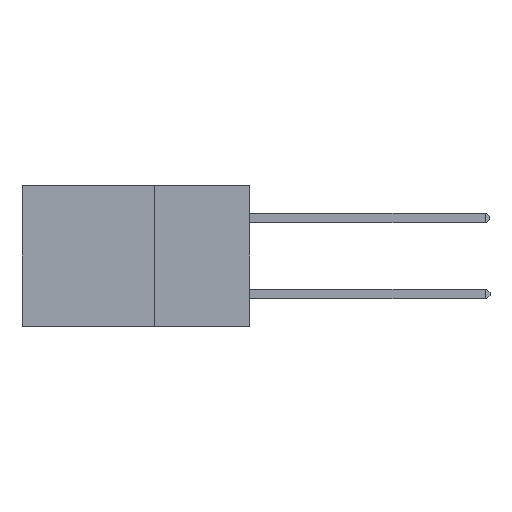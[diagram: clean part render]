
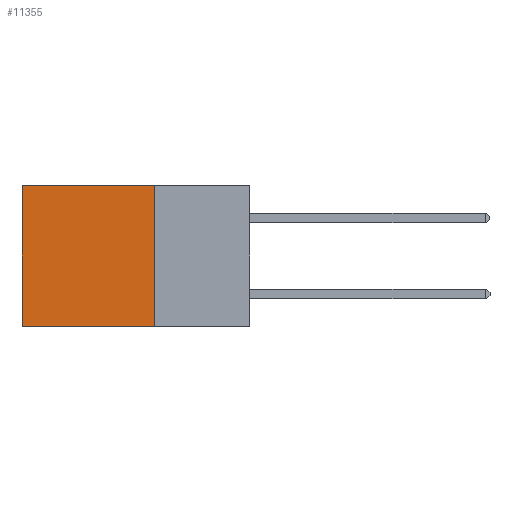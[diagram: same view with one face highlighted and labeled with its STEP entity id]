
A CAD part, left-side view. The second image highlights one B-rep face of the part: STEP entity #11355.
In plain terms, the highlighted planar face has unit normal (-1, 0, 0).
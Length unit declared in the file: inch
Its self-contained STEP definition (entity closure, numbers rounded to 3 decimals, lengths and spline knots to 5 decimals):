
#201 = CARTESIAN_POINT ( 'NONE',  ( 0.2875, 0.25, 0. ) ) ;
#1177 = CARTESIAN_POINT ( 'NONE',  ( 0.2875, 0.6, -0.37 ) ) ;
#2882 = VERTEX_POINT ( 'NONE', #5942 ) ;
#3474 = PLANE ( 'NONE',  #15855 ) ;
#3549 = VERTEX_POINT ( 'NONE', #1177 ) ;
#3553 = DIRECTION ( 'NONE',  ( 0., 0., -1. ) ) ;
#5105 = VECTOR ( 'NONE', #10933, 39.37008 ) ;
#5109 = DIRECTION ( 'NONE',  ( 0., 1., 0. ) ) ;
#5942 = CARTESIAN_POINT ( 'NONE',  ( 0.2875, 0.6, 0. ) ) ;
#6103 = CARTESIAN_POINT ( 'NONE',  ( 0.2875, 0.6, 0. ) ) ;
#8632 = CARTESIAN_POINT ( 'NONE',  ( 0.2875, 0.25, -0.37 ) ) ;
#9054 = DIRECTION ( 'NONE',  ( 0., 0., -1. ) ) ;
#9189 = CARTESIAN_POINT ( 'NONE',  ( 0.2875, 0.25, 0. ) ) ;
#10525 = CARTESIAN_POINT ( 'NONE',  ( 0.2875, 0.25, 0. ) ) ;
#10740 = LINE ( 'NONE', #6103, #14750 ) ;
#10933 = DIRECTION ( 'NONE',  ( 0., 1., 0. ) ) ;
#11355 = ADVANCED_FACE ( 'NONE', ( #15709 ), #3474, .F. ) ;
#11740 = VECTOR ( 'NONE', #5109, 39.37008 ) ;
#11860 = VERTEX_POINT ( 'NONE', #22137 ) ;
#12883 = CARTESIAN_POINT ( 'NONE',  ( 0.2875, 0.25, 0. ) ) ;
#13973 = DIRECTION ( 'NONE',  ( 1., 0., 0. ) ) ;
#14294 = LINE ( 'NONE', #9189, #5105 ) ;
#14386 = ORIENTED_EDGE ( 'NONE', *, *, #21253, .T. ) ;
#14602 = EDGE_CURVE ( 'NONE', #2882, #3549, #10740, .T. ) ;
#14750 = VECTOR ( 'NONE', #21590, 39.37008 ) ;
#15709 = FACE_OUTER_BOUND ( 'NONE', #16225, .T. ) ;
#15855 = AXIS2_PLACEMENT_3D ( 'NONE', #10525, #13973, #3553 ) ;
#16218 = EDGE_CURVE ( 'NONE', #11860, #3549, #19812, .T. ) ;
#16223 = VECTOR ( 'NONE', #9054, 39.37008 ) ;
#16225 = EDGE_LOOP ( 'NONE', ( #18438, #16562, #20366, #14386 ) ) ;
#16562 = ORIENTED_EDGE ( 'NONE', *, *, #16218, .F. ) ;
#18438 = ORIENTED_EDGE ( 'NONE', *, *, #14602, .T. ) ;
#19812 = LINE ( 'NONE', #8632, #11740 ) ;
#20366 = ORIENTED_EDGE ( 'NONE', *, *, #21347, .F. ) ;
#20786 = LINE ( 'NONE', #201, #16223 ) ;
#21253 = EDGE_CURVE ( 'NONE', #22188, #2882, #14294, .T. ) ;
#21347 = EDGE_CURVE ( 'NONE', #22188, #11860, #20786, .T. ) ;
#21590 = DIRECTION ( 'NONE',  ( 0., 0., -1. ) ) ;
#22137 = CARTESIAN_POINT ( 'NONE',  ( 0.2875, 0.25, -0.37 ) ) ;
#22188 = VERTEX_POINT ( 'NONE', #12883 ) ;
